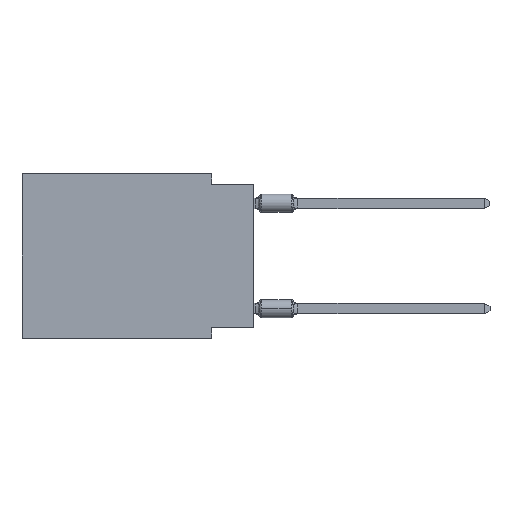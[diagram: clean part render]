
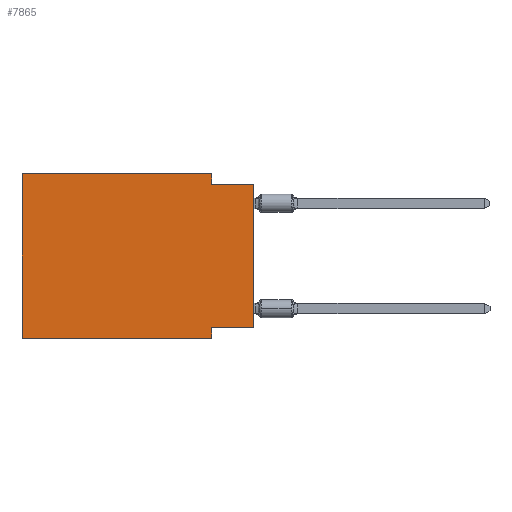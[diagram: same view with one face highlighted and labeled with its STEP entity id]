
A CAD part, left-side view. The second image highlights one B-rep face of the part: STEP entity #7865.
In plain terms, the highlighted planar face has unit normal (-1, 0, 0).
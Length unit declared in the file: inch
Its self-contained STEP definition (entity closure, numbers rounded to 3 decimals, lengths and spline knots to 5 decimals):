
#118 = DIRECTION ( 'NONE',  ( 1., 0., 0. ) ) ;
#137 = DIRECTION ( 'NONE',  ( 0., -1., 0. ) ) ;
#194 = EDGE_CURVE ( 'NONE', #7142, #15637, #7567, .T. ) ;
#368 = CARTESIAN_POINT ( 'NONE',  ( 0., 0.55, -0.39 ) ) ;
#404 = VERTEX_POINT ( 'NONE', #13888 ) ;
#645 = ORIENTED_EDGE ( 'NONE', *, *, #690, .T. ) ;
#690 = EDGE_CURVE ( 'NONE', #4632, #2209, #5149, .T. ) ;
#922 = VECTOR ( 'NONE', #3843, 39.37008 ) ;
#1344 = CARTESIAN_POINT ( 'NONE',  ( 0., 0.55, 0. ) ) ;
#1702 = ORIENTED_EDGE ( 'NONE', *, *, #194, .F. ) ;
#1765 = ORIENTED_EDGE ( 'NONE', *, *, #6158, .F. ) ;
#1786 = VECTOR ( 'NONE', #14065, 39.37008 ) ;
#1880 = VECTOR ( 'NONE', #7547, 39.37008 ) ;
#2082 = VECTOR ( 'NONE', #15105, 39.37008 ) ;
#2209 = VERTEX_POINT ( 'NONE', #15416 ) ;
#2510 = PLANE ( 'NONE',  #10881 ) ;
#2625 = ORIENTED_EDGE ( 'NONE', *, *, #10226, .F. ) ;
#2835 = EDGE_CURVE ( 'NONE', #10462, #14202, #14835, .T. ) ;
#3095 = CARTESIAN_POINT ( 'NONE',  ( 0., 0.1, -0.39 ) ) ;
#3262 = ORIENTED_EDGE ( 'NONE', *, *, #2835, .T. ) ;
#3498 = VECTOR ( 'NONE', #137, 39.37008 ) ;
#3538 = VERTEX_POINT ( 'NONE', #11121 ) ;
#3793 = LINE ( 'NONE', #9712, #3498 ) ;
#3843 = DIRECTION ( 'NONE',  ( 0., 0., 1. ) ) ;
#4202 = DIRECTION ( 'NONE',  ( 0., 0., -1. ) ) ;
#4304 = LINE ( 'NONE', #9188, #1786 ) ;
#4519 = ORIENTED_EDGE ( 'NONE', *, *, #13718, .F. ) ;
#4632 = VERTEX_POINT ( 'NONE', #5775 ) ;
#5113 = CARTESIAN_POINT ( 'NONE',  ( 0., 0.55, 0. ) ) ;
#5149 = LINE ( 'NONE', #368, #1880 ) ;
#5180 = VECTOR ( 'NONE', #6200, 39.37008 ) ;
#5428 = EDGE_CURVE ( 'NONE', #4632, #7142, #9926, .T. ) ;
#5507 = VECTOR ( 'NONE', #4202, 39.37008 ) ;
#5775 = CARTESIAN_POINT ( 'NONE',  ( 0., 0.55, -0.39 ) ) ;
#5948 = EDGE_CURVE ( 'NONE', #3538, #2209, #6606, .T. ) ;
#6125 = CARTESIAN_POINT ( 'NONE',  ( 0., 0.1, 0. ) ) ;
#6158 = EDGE_CURVE ( 'NONE', #404, #14202, #3793, .T. ) ;
#6200 = DIRECTION ( 'NONE',  ( 0., -1., 0. ) ) ;
#6606 = LINE ( 'NONE', #3095, #5507 ) ;
#7142 = VERTEX_POINT ( 'NONE', #5113 ) ;
#7372 = DIRECTION ( 'NONE',  ( 0., 0., -1. ) ) ;
#7547 = DIRECTION ( 'NONE',  ( 0., -1., 0. ) ) ;
#7567 = LINE ( 'NONE', #1344, #5180 ) ;
#7865 = ADVANCED_FACE ( 'NONE', ( #13524 ), #2510, .F. ) ;
#8651 = CARTESIAN_POINT ( 'NONE',  ( 0., 0.55, 0. ) ) ;
#9062 = ORIENTED_EDGE ( 'NONE', *, *, #5428, .F. ) ;
#9188 = CARTESIAN_POINT ( 'NONE',  ( 0., 0.1, 0. ) ) ;
#9628 = EDGE_LOOP ( 'NONE', ( #3262, #1765, #2625, #1702, #9062, #645, #11342, #4519 ) ) ;
#9661 = CARTESIAN_POINT ( 'NONE',  ( 0., 0., -0.365 ) ) ;
#9712 = CARTESIAN_POINT ( 'NONE',  ( 0., 0., -0.025 ) ) ;
#9926 = LINE ( 'NONE', #14793, #922 ) ;
#10226 = EDGE_CURVE ( 'NONE', #15637, #404, #4304, .T. ) ;
#10462 = VERTEX_POINT ( 'NONE', #9661 ) ;
#10881 = AXIS2_PLACEMENT_3D ( 'NONE', #8651, #118, #7372 ) ;
#11121 = CARTESIAN_POINT ( 'NONE',  ( 0., 0.1, -0.365 ) ) ;
#11198 = LINE ( 'NONE', #14792, #2082 ) ;
#11342 = ORIENTED_EDGE ( 'NONE', *, *, #5948, .F. ) ;
#12336 = VECTOR ( 'NONE', #14913, 39.37008 ) ;
#12612 = CARTESIAN_POINT ( 'NONE',  ( 0., 0., 0. ) ) ;
#13524 = FACE_OUTER_BOUND ( 'NONE', #9628, .T. ) ;
#13718 = EDGE_CURVE ( 'NONE', #10462, #3538, #11198, .T. ) ;
#13888 = CARTESIAN_POINT ( 'NONE',  ( 0., 0.1, -0.025 ) ) ;
#14065 = DIRECTION ( 'NONE',  ( 0., 0., -1. ) ) ;
#14202 = VERTEX_POINT ( 'NONE', #15011 ) ;
#14792 = CARTESIAN_POINT ( 'NONE',  ( 0., 0., -0.365 ) ) ;
#14793 = CARTESIAN_POINT ( 'NONE',  ( 0., 0.55, 0. ) ) ;
#14835 = LINE ( 'NONE', #12612, #12336 ) ;
#14913 = DIRECTION ( 'NONE',  ( 0., 0., 1. ) ) ;
#15011 = CARTESIAN_POINT ( 'NONE',  ( 0., 0., -0.025 ) ) ;
#15105 = DIRECTION ( 'NONE',  ( 0., 1., 0. ) ) ;
#15416 = CARTESIAN_POINT ( 'NONE',  ( 0., 0.1, -0.39 ) ) ;
#15637 = VERTEX_POINT ( 'NONE', #6125 ) ;
